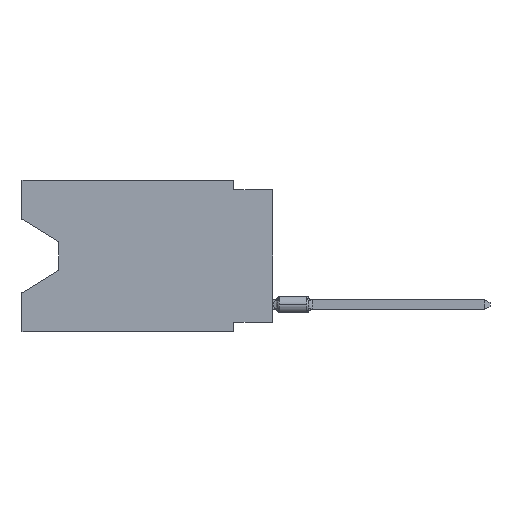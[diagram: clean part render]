
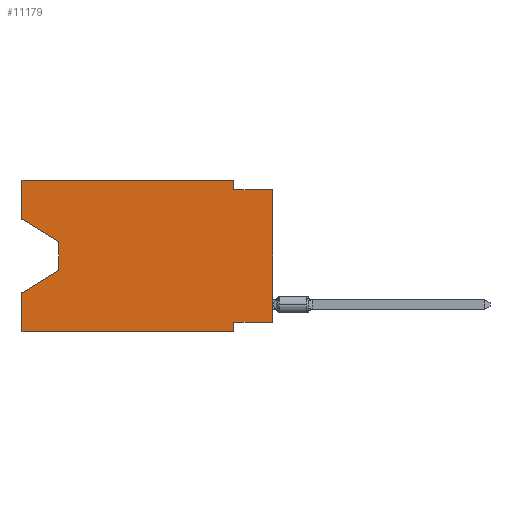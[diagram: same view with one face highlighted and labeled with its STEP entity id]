
A CAD part, left-side view. The second image highlights one B-rep face of the part: STEP entity #11179.
In plain terms, the highlighted planar face has unit normal (-1, 0, 0).
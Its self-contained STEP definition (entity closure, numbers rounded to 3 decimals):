
#436 = DIRECTION ( 'NONE',  ( 0., 0., -1. ) ) ;
#926 = CARTESIAN_POINT ( 'NONE',  ( 0., 2.54, -9.906 ) ) ;
#974 = CARTESIAN_POINT ( 'NONE',  ( 0., 16.383, 0. ) ) ;
#1068 = EDGE_CURVE ( 'NONE', #7212, #29020, #14137, .T. ) ;
#1511 = CARTESIAN_POINT ( 'NONE',  ( 0., 16.383, -2.546 ) ) ;
#2698 = CARTESIAN_POINT ( 'NONE',  ( 0., 16.383, -9.906 ) ) ;
#2920 = EDGE_CURVE ( 'NONE', #14043, #11726, #3676, .T. ) ;
#2939 = VERTEX_POINT ( 'NONE', #13477 ) ;
#3265 = VERTEX_POINT ( 'NONE', #13588 ) ;
#3352 = ORIENTED_EDGE ( 'NONE', *, *, #20845, .F. ) ;
#3676 = LINE ( 'NONE', #5536, #24869 ) ;
#3866 = CARTESIAN_POINT ( 'NONE',  ( 0., 2.54, -9.906 ) ) ;
#4083 = EDGE_CURVE ( 'NONE', #12094, #3265, #10982, .T. ) ;
#4382 = CARTESIAN_POINT ( 'NONE',  ( 0., 2.54, -9.271 ) ) ;
#4900 = EDGE_CURVE ( 'NONE', #13184, #2939, #32311, .T. ) ;
#5145 = AXIS2_PLACEMENT_3D ( 'NONE', #974, #21379, #18850 ) ;
#5393 = ORIENTED_EDGE ( 'NONE', *, *, #8650, .F. ) ;
#5536 = CARTESIAN_POINT ( 'NONE',  ( 0., 13.97, -4.013 ) ) ;
#5853 = ORIENTED_EDGE ( 'NONE', *, *, #7565, .F. ) ;
#6164 = VERTEX_POINT ( 'NONE', #24068 ) ;
#6268 = CARTESIAN_POINT ( 'NONE',  ( 0., 16.383, 0. ) ) ;
#6891 = LINE ( 'NONE', #3866, #9968 ) ;
#7212 = VERTEX_POINT ( 'NONE', #26547 ) ;
#7260 = DIRECTION ( 'NONE',  ( 0., -1., 0. ) ) ;
#7498 = LINE ( 'NONE', #17787, #27255 ) ;
#7565 = EDGE_CURVE ( 'NONE', #6164, #12094, #32082, .T. ) ;
#7669 = ORIENTED_EDGE ( 'NONE', *, *, #19481, .F. ) ;
#7761 = LINE ( 'NONE', #2698, #33132 ) ;
#7948 = CARTESIAN_POINT ( 'NONE',  ( 0., 16.383, 0. ) ) ;
#8650 = EDGE_CURVE ( 'NONE', #3265, #31432, #12247, .T. ) ;
#8969 = DIRECTION ( 'NONE',  ( 0., 0., 1. ) ) ;
#9724 = ORIENTED_EDGE ( 'NONE', *, *, #4083, .F. ) ;
#9968 = VECTOR ( 'NONE', #29358, 1000. ) ;
#10048 = EDGE_CURVE ( 'NONE', #6164, #14043, #24630, .T. ) ;
#10118 = DIRECTION ( 'NONE',  ( 0., -1., 0. ) ) ;
#10225 = DIRECTION ( 'NONE',  ( 0., 1., 0. ) ) ;
#10923 = FACE_OUTER_BOUND ( 'NONE', #30801, .T. ) ;
#10982 = LINE ( 'NONE', #7948, #32470 ) ;
#11107 = DIRECTION ( 'NONE',  ( 0., 0., -1. ) ) ;
#11179 = ADVANCED_FACE ( 'NONE', ( #10923 ), #19014, .F. ) ;
#11726 = VERTEX_POINT ( 'NONE', #13917 ) ;
#11986 = LINE ( 'NONE', #32890, #30239 ) ;
#12094 = VERTEX_POINT ( 'NONE', #32624 ) ;
#12247 = LINE ( 'NONE', #18295, #14286 ) ;
#12607 = VECTOR ( 'NONE', #8969, 1000. ) ;
#12774 = CARTESIAN_POINT ( 'NONE',  ( 0., 13.97, -4.013 ) ) ;
#13184 = VERTEX_POINT ( 'NONE', #16830 ) ;
#13477 = CARTESIAN_POINT ( 'NONE',  ( 0., 16.383, -7.36 ) ) ;
#13513 = DIRECTION ( 'NONE',  ( 0., -1., 0. ) ) ;
#13588 = CARTESIAN_POINT ( 'NONE',  ( 0., 2.54, 0. ) ) ;
#13805 = EDGE_CURVE ( 'NONE', #11726, #2939, #7498, .T. ) ;
#13917 = CARTESIAN_POINT ( 'NONE',  ( 0., 13.97, -5.893 ) ) ;
#14043 = VERTEX_POINT ( 'NONE', #12774 ) ;
#14091 = CARTESIAN_POINT ( 'NONE',  ( 0., 16.383, 0. ) ) ;
#14137 = LINE ( 'NONE', #25579, #18950 ) ;
#14286 = VECTOR ( 'NONE', #436, 1000. ) ;
#14794 = VECTOR ( 'NONE', #30334, 1000. ) ;
#16830 = CARTESIAN_POINT ( 'NONE',  ( 0., 16.383, -9.906 ) ) ;
#17787 = CARTESIAN_POINT ( 'NONE',  ( 0., 13.97, -5.893 ) ) ;
#17954 = DIRECTION ( 'NONE',  ( 0., 0.855, -0.519 ) ) ;
#18295 = CARTESIAN_POINT ( 'NONE',  ( 0., 2.54, 0. ) ) ;
#18850 = DIRECTION ( 'NONE',  ( 0., 0., -1. ) ) ;
#18950 = VECTOR ( 'NONE', #10225, 1000. ) ;
#18994 = ORIENTED_EDGE ( 'NONE', *, *, #2920, .T. ) ;
#19014 = PLANE ( 'NONE',  #5145 ) ;
#19481 = EDGE_CURVE ( 'NONE', #31432, #26855, #11986, .T. ) ;
#19979 = ORIENTED_EDGE ( 'NONE', *, *, #1068, .F. ) ;
#20022 = VERTEX_POINT ( 'NONE', #926 ) ;
#20641 = EDGE_CURVE ( 'NONE', #13184, #20022, #7761, .T. ) ;
#20785 = ORIENTED_EDGE ( 'NONE', *, *, #10048, .T. ) ;
#20845 = EDGE_CURVE ( 'NONE', #29020, #20022, #6891, .T. ) ;
#21379 = DIRECTION ( 'NONE',  ( 1., 0., 0. ) ) ;
#21865 = EDGE_CURVE ( 'NONE', #7212, #26855, #26511, .T. ) ;
#23452 = ORIENTED_EDGE ( 'NONE', *, *, #21865, .T. ) ;
#24068 = CARTESIAN_POINT ( 'NONE',  ( 0., 16.383, -2.546 ) ) ;
#24245 = CARTESIAN_POINT ( 'NONE',  ( 0., 2.54, -0.635 ) ) ;
#24475 = CARTESIAN_POINT ( 'NONE',  ( 0., 0., 0. ) ) ;
#24630 = LINE ( 'NONE', #1511, #14794 ) ;
#24869 = VECTOR ( 'NONE', #11107, 1000. ) ;
#25579 = CARTESIAN_POINT ( 'NONE',  ( 0., 0., -9.271 ) ) ;
#26511 = LINE ( 'NONE', #24475, #32523 ) ;
#26547 = CARTESIAN_POINT ( 'NONE',  ( 0., 0., -9.271 ) ) ;
#26855 = VERTEX_POINT ( 'NONE', #29582 ) ;
#27255 = VECTOR ( 'NONE', #17954, 1000. ) ;
#29020 = VERTEX_POINT ( 'NONE', #4382 ) ;
#29119 = DIRECTION ( 'NONE',  ( 0., 0., 1. ) ) ;
#29334 = ORIENTED_EDGE ( 'NONE', *, *, #4900, .F. ) ;
#29358 = DIRECTION ( 'NONE',  ( 0., 0., -1. ) ) ;
#29548 = ORIENTED_EDGE ( 'NONE', *, *, #20641, .T. ) ;
#29549 = DIRECTION ( 'NONE',  ( 0., 0., 1. ) ) ;
#29582 = CARTESIAN_POINT ( 'NONE',  ( 0., 0., -0.635 ) ) ;
#30133 = VECTOR ( 'NONE', #29119, 1000. ) ;
#30239 = VECTOR ( 'NONE', #10118, 1000. ) ;
#30334 = DIRECTION ( 'NONE',  ( 0., -0.855, -0.519 ) ) ;
#30801 = EDGE_LOOP ( 'NONE', ( #20785, #18994, #32055, #29334, #29548, #3352, #19979, #23452, #7669, #5393, #9724, #5853 ) ) ;
#31432 = VERTEX_POINT ( 'NONE', #24245 ) ;
#32055 = ORIENTED_EDGE ( 'NONE', *, *, #13805, .T. ) ;
#32082 = LINE ( 'NONE', #6268, #12607 ) ;
#32311 = LINE ( 'NONE', #14091, #30133 ) ;
#32470 = VECTOR ( 'NONE', #13513, 1000. ) ;
#32523 = VECTOR ( 'NONE', #29549, 1000. ) ;
#32624 = CARTESIAN_POINT ( 'NONE',  ( 0., 16.383, 0. ) ) ;
#32890 = CARTESIAN_POINT ( 'NONE',  ( 0., 0., -0.635 ) ) ;
#33132 = VECTOR ( 'NONE', #7260, 1000. ) ;
